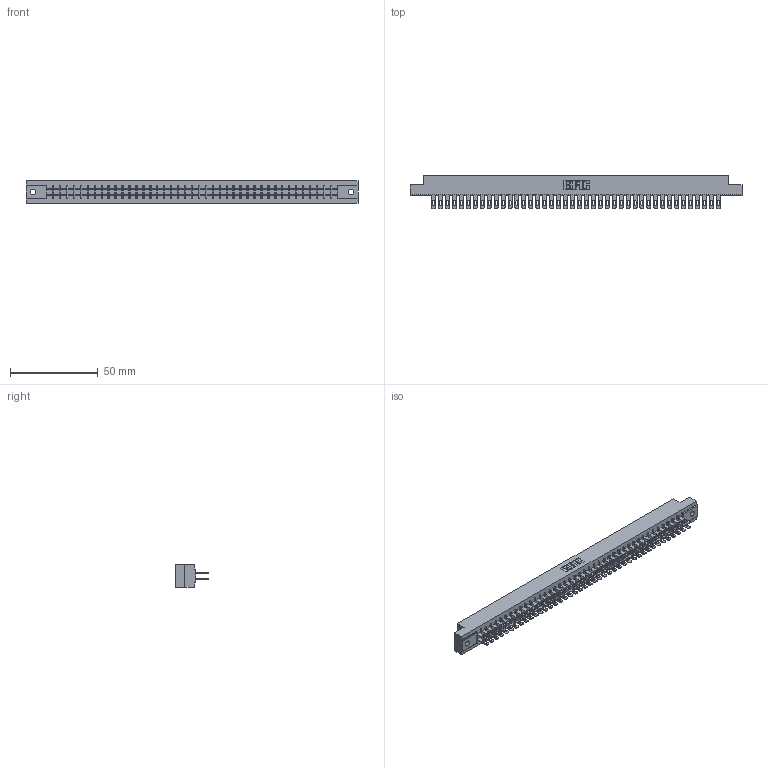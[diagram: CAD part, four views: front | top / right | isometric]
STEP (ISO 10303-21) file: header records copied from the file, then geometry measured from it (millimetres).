
FILE_DESCRIPTION (( 'STEP AP203' ), '1' );
FILE_NAME ('305-084-500-502.STEP', '2019-09-10T11:47:16', ( '' ), ( '' ), 'SwSTEP 2.0', 'SolidWorks 2016', '' );
FILE_SCHEMA (( 'CONFIG_CONTROL_DESIGN' ));
Length unit declared in the file: inch
Products named in the file (3): 305-290-001_500; 305-084-500-502; 305 Part_.128 Dia
Assembly tree (85 placements, depth 2):
  305-084-500-502
    305 Part_.128 Dia
    305-290-001_500  x84
Bounding box: 189.43 x 18.85 x 12.7 mm (x, y, z)
Volume: 19405 mm3; surface area: 26989.8 mm2
Topology: 85 solids, 85 shells, 4316 faces, 12370 edges, 8020 vertices
Faces by surface type: plane 2420, cylinder 1728, sphere 168
Entity records: 45499 total; most frequent: CARTESIAN_POINT 7528, ORIENTED_EDGE 7472, DIRECTION 7284, EDGE_CURVE 3736, VECTOR 3020, LINE 3020, VERTEX_POINT 2376, AXIS2_PLACEMENT_3D 2132
